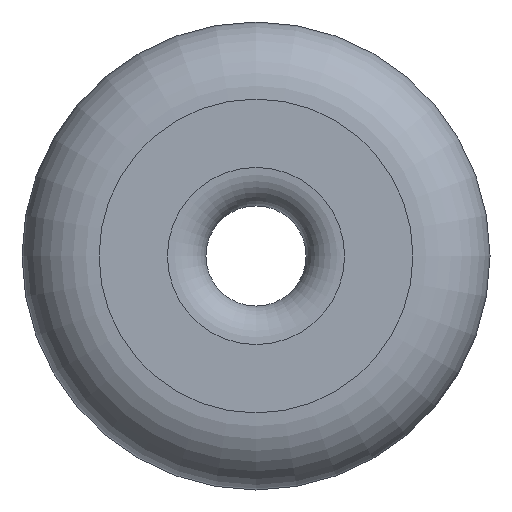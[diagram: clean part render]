
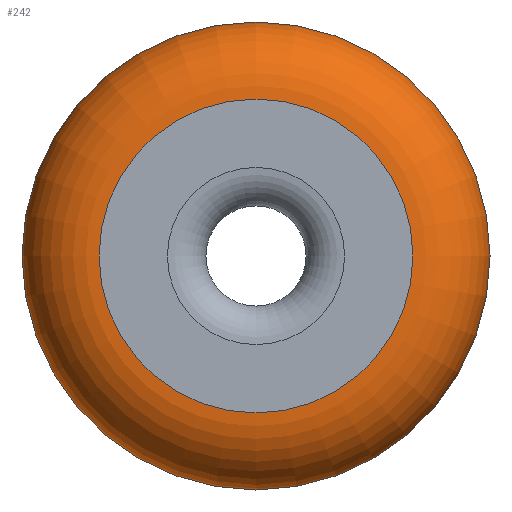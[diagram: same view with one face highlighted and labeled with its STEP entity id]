
A CAD part, front view. The second image highlights one B-rep face of the part: STEP entity #242.
In plain terms, the highlighted toroidal (fillet/blend) face has major radius 15.519 mm and minor radius 7.62 mm.
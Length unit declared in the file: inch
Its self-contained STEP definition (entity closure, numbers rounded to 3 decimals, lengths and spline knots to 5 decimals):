
#188=CARTESIAN_POINT('',(0.611,-5.9,0.0));
#189=VERTEX_POINT('',#188);
#190=CARTESIAN_POINT('',(0.0,-5.9,0.0));
#191=DIRECTION('',(0.0,1.0,0.0));
#192=DIRECTION('',(-1.0,0.0,0.0));
#193=AXIS2_PLACEMENT_3D('',#190,#191,#192);
#194=CIRCLE('',#193,0.611);
#195=EDGE_CURVE('',#189,#189,#194,.T.);
#223=CARTESIAN_POINT('',(0.0,-5.6,0.0));
#224=DIRECTION('',(0.0,1.0,0.0));
#225=DIRECTION('',(0.0,0.0,1.0));
#226=AXIS2_PLACEMENT_3D('',#223,#224,#225);
#227=TOROIDAL_SURFACE('',#226,0.611,0.3);
#228=ORIENTED_EDGE('',*,*,#195,.T.);
#229=EDGE_LOOP('',(#228));
#230=FACE_OUTER_BOUND('',#229,.T.);
#231=CARTESIAN_POINT('',(0.911,-5.6,0.));
#232=VERTEX_POINT('',#231);
#233=CARTESIAN_POINT('',(0.0,-5.6,0.0));
#234=DIRECTION('',(0.0,-1.0,0.0));
#235=DIRECTION('',(-1.0,0.0,0.0));
#236=AXIS2_PLACEMENT_3D('',#233,#234,#235);
#237=CIRCLE('',#236,0.911);
#238=EDGE_CURVE('',#232,#232,#237,.T.);
#239=ORIENTED_EDGE('',*,*,#238,.T.);
#240=EDGE_LOOP('',(#239));
#241=FACE_BOUND('',#240,.T.);
#242=ADVANCED_FACE('',(#230,#241),#227,.T.);
